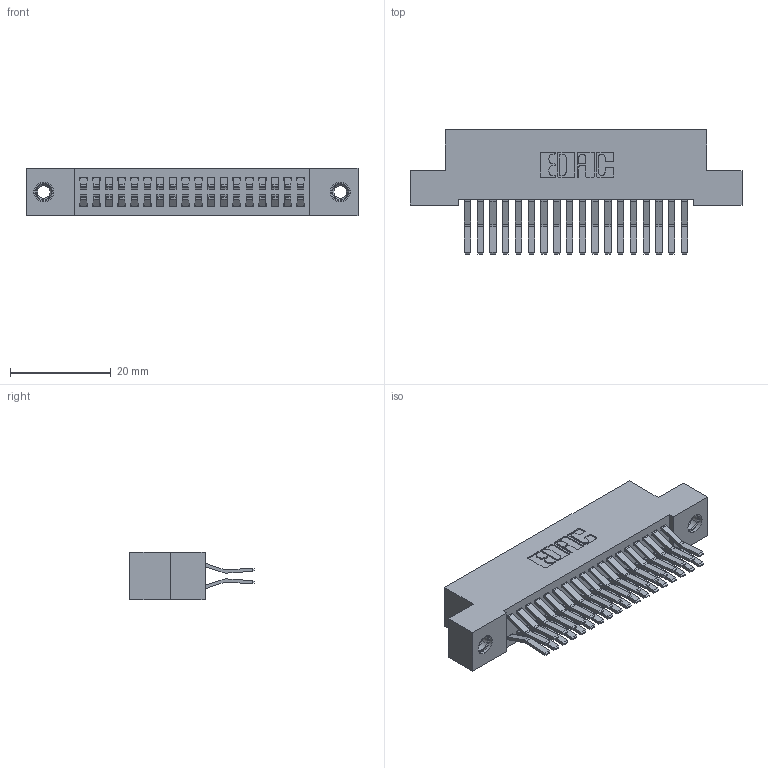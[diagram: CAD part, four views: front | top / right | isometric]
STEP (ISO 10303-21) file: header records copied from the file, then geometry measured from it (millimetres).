
FILE_DESCRIPTION (( 'STEP AP203' ), '1' );
FILE_NAME ('392-036-560-207.STEP', '2019-10-07T17:46:59', ( '' ), ( '' ), 'SwSTEP 2.0', 'SolidWorks 2016', '' );
FILE_SCHEMA (( 'CONFIG_CONTROL_DESIGN' ));
Length unit declared in the file: inch
Products named in the file (4): 345-292-001_560 Tail; 345-250-001_345-250-005-103; 392-036-560-207; 342 Part_TI
Assembly tree (39 placements, depth 2):
  392-036-560-207
    342 Part_TI
    345-292-001_560 Tail  x36
    345-250-001_345-250-005-103  x2
Bounding box: 66.04 x 24.78 x 9.4 mm (x, y, z)
Volume: 6043.8 mm3; surface area: 9838.9 mm2
Topology: 39 solids, 39 shells, 2114 faces, 6231 edges, 4098 vertices
Faces by surface type: plane 1394, cylinder 704, cone 12, torus 4
Entity records: 15826 total; most frequent: CARTESIAN_POINT 2633, ORIENTED_EDGE 2562, DIRECTION 2327, EDGE_CURVE 1281, LINE 1129, VECTOR 1129, VERTEX_POINT 848, AXIS2_PLACEMENT_3D 599
